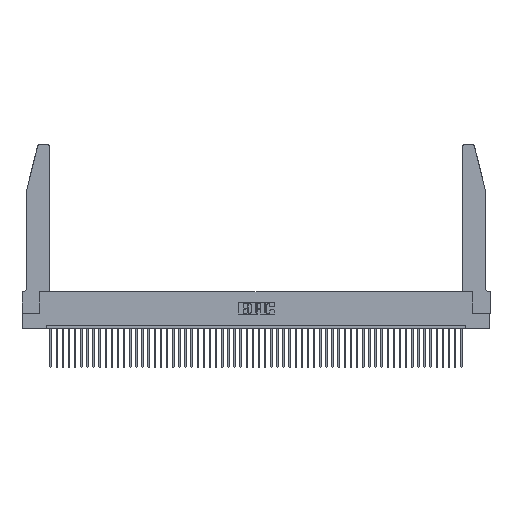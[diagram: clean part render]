
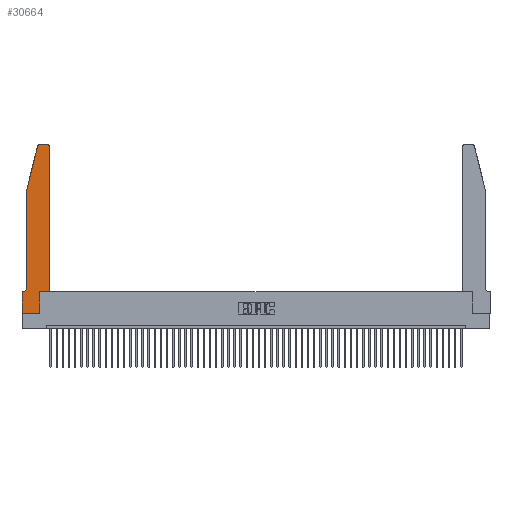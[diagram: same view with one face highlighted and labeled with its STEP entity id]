
A CAD part, top view. The second image highlights one B-rep face of the part: STEP entity #30664.
In plain terms, the highlighted planar face has unit normal (0, 0, 1).
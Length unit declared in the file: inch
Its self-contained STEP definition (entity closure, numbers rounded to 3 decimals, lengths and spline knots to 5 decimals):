
#64 = CARTESIAN_POINT ( 'NONE',  ( 0., 0., 0.37 ) ) ;
#340 = CIRCLE ( 'NONE', #31235, 0.07 ) ;
#393 = EDGE_CURVE ( 'NONE', #46995, #709, #24508, .T. ) ;
#534 = EDGE_CURVE ( 'NONE', #4650, #31667, #340, .T. ) ;
#545 = DIRECTION ( 'NONE',  ( 0., 0., -1. ) ) ;
#709 = VERTEX_POINT ( 'NONE', #21766 ) ;
#1640 = VERTEX_POINT ( 'NONE', #49030 ) ;
#1951 = ORIENTED_EDGE ( 'NONE', *, *, #40974, .T. ) ;
#2024 = VECTOR ( 'NONE', #14701, 39.37008 ) ;
#2901 = EDGE_CURVE ( 'NONE', #35752, #46995, #19802, .T. ) ;
#3363 = DIRECTION ( 'NONE',  ( 0., 1., 0. ) ) ;
#3932 = DIRECTION ( 'NONE',  ( -0.239, -0.971, 0. ) ) ;
#4650 = VERTEX_POINT ( 'NONE', #15660 ) ;
#5438 = VECTOR ( 'NONE', #3932, 39.37008 ) ;
#6773 = CARTESIAN_POINT ( 'NONE',  ( 0., 0.35, 0.37 ) ) ;
#7651 = EDGE_CURVE ( 'NONE', #31667, #8493, #20989, .T. ) ;
#8493 = VERTEX_POINT ( 'NONE', #6773 ) ;
#9228 = CARTESIAN_POINT ( 'NONE',  ( 0., 0.35, 0.37 ) ) ;
#9355 = ORIENTED_EDGE ( 'NONE', *, *, #7651, .T. ) ;
#9858 = VECTOR ( 'NONE', #11418, 39.37008 ) ;
#10566 = DIRECTION ( 'NONE',  ( -1., 0., 0. ) ) ;
#10607 = AXIS2_PLACEMENT_3D ( 'NONE', #48757, #26498, #43593 ) ;
#10958 = EDGE_CURVE ( 'NONE', #18182, #4650, #34484, .T. ) ;
#11081 = CARTESIAN_POINT ( 'NONE',  ( 0.4505, 2.72, 0.37 ) ) ;
#11121 = CARTESIAN_POINT ( 'NONE',  ( 0.0755, 2., 0.37 ) ) ;
#11418 = DIRECTION ( 'NONE',  ( 0., -1., 0. ) ) ;
#11460 = CARTESIAN_POINT ( 'NONE',  ( 0.2865, 0.35, 0.37 ) ) ;
#11723 = LINE ( 'NONE', #24068, #20489 ) ;
#11751 = EDGE_CURVE ( 'NONE', #709, #19131, #11723, .T. ) ;
#11852 = DIRECTION ( 'NONE',  ( 1., 0., 0. ) ) ;
#13403 = VECTOR ( 'NONE', #32048, 39.37008 ) ;
#13870 = ORIENTED_EDGE ( 'NONE', *, *, #393, .T. ) ;
#14701 = DIRECTION ( 'NONE',  ( -1., 0., 0. ) ) ;
#15068 = ORIENTED_EDGE ( 'NONE', *, *, #10958, .T. ) ;
#15660 = CARTESIAN_POINT ( 'NONE',  ( 0.0755, 0.42, 0.37 ) ) ;
#16593 = FACE_OUTER_BOUND ( 'NONE', #28017, .T. ) ;
#16795 = DIRECTION ( 'NONE',  ( 1., 0., 0. ) ) ;
#18182 = VERTEX_POINT ( 'NONE', #11121 ) ;
#19131 = VERTEX_POINT ( 'NONE', #11081 ) ;
#19802 = LINE ( 'NONE', #24146, #13403 ) ;
#20489 = VECTOR ( 'NONE', #3363, 39.37008 ) ;
#20598 = CARTESIAN_POINT ( 'NONE',  ( 0.284, 2.75, 0.37 ) ) ;
#20989 = LINE ( 'NONE', #46882, #2024 ) ;
#21766 = CARTESIAN_POINT ( 'NONE',  ( 0.4505, 0.35, 0.37 ) ) ;
#21839 = ORIENTED_EDGE ( 'NONE', *, *, #2901, .T. ) ;
#22394 = CARTESIAN_POINT ( 'NONE',  ( 0., 0., 0.37 ) ) ;
#22595 = VECTOR ( 'NONE', #32795, 39.37008 ) ;
#23555 = VERTEX_POINT ( 'NONE', #20598 ) ;
#24068 = CARTESIAN_POINT ( 'NONE',  ( 0.4505, 0.35, 0.37 ) ) ;
#24095 = CARTESIAN_POINT ( 'NONE',  ( 0.0055, 0.42, 0.37 ) ) ;
#24146 = CARTESIAN_POINT ( 'NONE',  ( 0.2865, 0.35, 0.37 ) ) ;
#24508 = LINE ( 'NONE', #48609, #22595 ) ;
#24730 = EDGE_CURVE ( 'NONE', #38634, #18182, #32070, .T. ) ;
#24844 = CIRCLE ( 'NONE', #34476, 0.03 ) ;
#25743 = DIRECTION ( 'NONE',  ( 0., 0., 1. ) ) ;
#25949 = CIRCLE ( 'NONE', #10607, 0.03 ) ;
#26498 = DIRECTION ( 'NONE',  ( 0., 0., 1. ) ) ;
#26591 = CARTESIAN_POINT ( 'NONE',  ( 0., 0., 0.37 ) ) ;
#27620 = VECTOR ( 'NONE', #38856, 39.37008 ) ;
#28017 = EDGE_LOOP ( 'NONE', ( #35344, #29404, #28664, #15068, #45859, #9355, #1951, #41488, #21839, #13870, #32922, #37030 ) ) ;
#28584 = LINE ( 'NONE', #22394, #29145 ) ;
#28664 = ORIENTED_EDGE ( 'NONE', *, *, #24730, .T. ) ;
#29145 = VECTOR ( 'NONE', #46396, 39.37008 ) ;
#29312 = CARTESIAN_POINT ( 'NONE',  ( 0.2605, 2.75, 0.37 ) ) ;
#29404 = ORIENTED_EDGE ( 'NONE', *, *, #35256, .T. ) ;
#30664 = ADVANCED_FACE ( 'NONE', ( #16593 ), #49384, .T. ) ;
#31235 = AXIS2_PLACEMENT_3D ( 'NONE', #24095, #545, #10566 ) ;
#31667 = VERTEX_POINT ( 'NONE', #45612 ) ;
#31836 = DIRECTION ( 'NONE',  ( 0., 0., 1. ) ) ;
#32022 = CARTESIAN_POINT ( 'NONE',  ( 0.25487, 2.72718, 0.37 ) ) ;
#32048 = DIRECTION ( 'NONE',  ( 0., 1., 0. ) ) ;
#32070 = LINE ( 'NONE', #52062, #5438 ) ;
#32222 = EDGE_CURVE ( 'NONE', #19131, #1640, #24844, .T. ) ;
#32795 = DIRECTION ( 'NONE',  ( 1., 0., 0. ) ) ;
#32893 = DIRECTION ( 'NONE',  ( -1., 0., 0. ) ) ;
#32922 = ORIENTED_EDGE ( 'NONE', *, *, #11751, .T. ) ;
#34476 = AXIS2_PLACEMENT_3D ( 'NONE', #43831, #31836, #11852 ) ;
#34484 = LINE ( 'NONE', #39232, #27620 ) ;
#35256 = EDGE_CURVE ( 'NONE', #23555, #38634, #25949, .T. ) ;
#35344 = ORIENTED_EDGE ( 'NONE', *, *, #50073, .T. ) ;
#35752 = VERTEX_POINT ( 'NONE', #49886 ) ;
#36192 = LINE ( 'NONE', #29312, #37975 ) ;
#36813 = VERTEX_POINT ( 'NONE', #26591 ) ;
#37030 = ORIENTED_EDGE ( 'NONE', *, *, #32222, .T. ) ;
#37975 = VECTOR ( 'NONE', #32893, 39.37008 ) ;
#38634 = VERTEX_POINT ( 'NONE', #32022 ) ;
#38856 = DIRECTION ( 'NONE',  ( 0., -1., 0. ) ) ;
#39232 = CARTESIAN_POINT ( 'NONE',  ( 0.0755, 2., 0.37 ) ) ;
#40974 = EDGE_CURVE ( 'NONE', #8493, #36813, #47979, .T. ) ;
#41488 = ORIENTED_EDGE ( 'NONE', *, *, #49602, .T. ) ;
#41847 = AXIS2_PLACEMENT_3D ( 'NONE', #9228, #25743, #16795 ) ;
#43593 = DIRECTION ( 'NONE',  ( 1., 0., 0. ) ) ;
#43831 = CARTESIAN_POINT ( 'NONE',  ( 0.4205, 2.72, 0.37 ) ) ;
#45612 = CARTESIAN_POINT ( 'NONE',  ( 0.0055, 0.35, 0.37 ) ) ;
#45859 = ORIENTED_EDGE ( 'NONE', *, *, #534, .T. ) ;
#46396 = DIRECTION ( 'NONE',  ( 1., 0., 0. ) ) ;
#46882 = CARTESIAN_POINT ( 'NONE',  ( 0.0755, 0.35, 0.37 ) ) ;
#46995 = VERTEX_POINT ( 'NONE', #11460 ) ;
#47979 = LINE ( 'NONE', #64, #9858 ) ;
#48609 = CARTESIAN_POINT ( 'NONE',  ( 0.4505, 0.35, 0.37 ) ) ;
#48757 = CARTESIAN_POINT ( 'NONE',  ( 0.284, 2.72, 0.37 ) ) ;
#49030 = CARTESIAN_POINT ( 'NONE',  ( 0.4205, 2.75, 0.37 ) ) ;
#49384 = PLANE ( 'NONE',  #41847 ) ;
#49602 = EDGE_CURVE ( 'NONE', #36813, #35752, #28584, .T. ) ;
#49886 = CARTESIAN_POINT ( 'NONE',  ( 0.2865, 0., 0.37 ) ) ;
#50073 = EDGE_CURVE ( 'NONE', #1640, #23555, #36192, .T. ) ;
#52062 = CARTESIAN_POINT ( 'NONE',  ( 0.0755, 2., 0.37 ) ) ;
